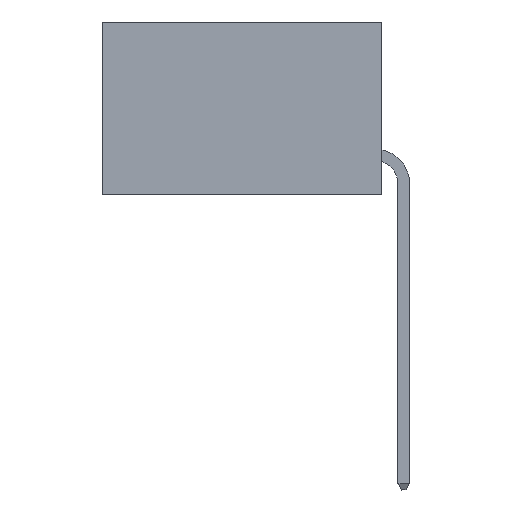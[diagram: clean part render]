
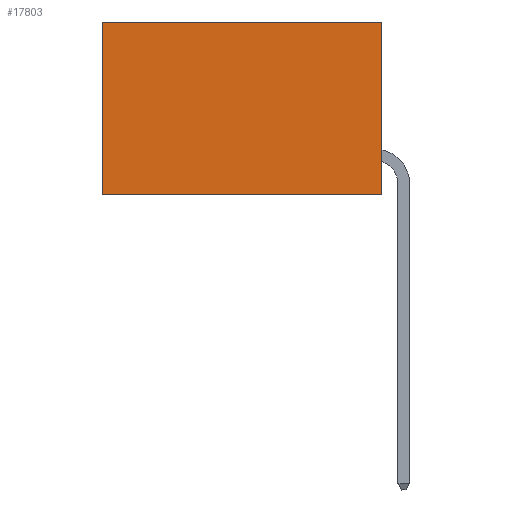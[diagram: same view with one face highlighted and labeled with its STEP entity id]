
A CAD part, left-side view. The second image highlights one B-rep face of the part: STEP entity #17803.
In plain terms, the highlighted planar face has unit normal (-1, 0, 0).
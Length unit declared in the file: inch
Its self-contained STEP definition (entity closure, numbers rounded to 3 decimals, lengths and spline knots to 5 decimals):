
#1202 = DIRECTION ( 'NONE',  ( 0., 0., -1. ) ) ;
#2442 = ORIENTED_EDGE ( 'NONE', *, *, #22988, .T. ) ;
#3109 = VERTEX_POINT ( 'NONE', #30400 ) ;
#3802 = CARTESIAN_POINT ( 'NONE',  ( 0.2875, 0., 0. ) ) ;
#4311 = VERTEX_POINT ( 'NONE', #10016 ) ;
#5636 = VECTOR ( 'NONE', #1202, 39.37008 ) ;
#6077 = ORIENTED_EDGE ( 'NONE', *, *, #27739, .F. ) ;
#6098 = VERTEX_POINT ( 'NONE', #28958 ) ;
#6115 = CARTESIAN_POINT ( 'NONE',  ( 0.2875, 0., 0. ) ) ;
#7193 = DIRECTION ( 'NONE',  ( 0., 0., -1. ) ) ;
#7658 = PLANE ( 'NONE',  #11790 ) ;
#7664 = EDGE_CURVE ( 'NONE', #16431, #3109, #23859, .T. ) ;
#9988 = ORIENTED_EDGE ( 'NONE', *, *, #7664, .T. ) ;
#10016 = CARTESIAN_POINT ( 'NONE',  ( 0.2875, 0., -0.37 ) ) ;
#10229 = DIRECTION ( 'NONE',  ( 0., 1., 0. ) ) ;
#10330 = CARTESIAN_POINT ( 'NONE',  ( 0.2875, 0., 0. ) ) ;
#10453 = EDGE_CURVE ( 'NONE', #16431, #4311, #30232, .T. ) ;
#10550 = ORIENTED_EDGE ( 'NONE', *, *, #10453, .F. ) ;
#11790 = AXIS2_PLACEMENT_3D ( 'NONE', #10330, #23190, #7193 ) ;
#11953 = VECTOR ( 'NONE', #15576, 39.37008 ) ;
#12030 = EDGE_LOOP ( 'NONE', ( #2442, #6077, #10550, #9988 ) ) ;
#12722 = CARTESIAN_POINT ( 'NONE',  ( 0.2875, 0., 0. ) ) ;
#15065 = VECTOR ( 'NONE', #10229, 39.37008 ) ;
#15576 = DIRECTION ( 'NONE',  ( 0., 0., -1. ) ) ;
#16431 = VERTEX_POINT ( 'NONE', #12722 ) ;
#17803 = ADVANCED_FACE ( 'NONE', ( #21502 ), #7658, .F. ) ;
#19664 = VECTOR ( 'NONE', #22470, 39.37008 ) ;
#21502 = FACE_OUTER_BOUND ( 'NONE', #12030, .T. ) ;
#22470 = DIRECTION ( 'NONE',  ( 0., 1., 0. ) ) ;
#22988 = EDGE_CURVE ( 'NONE', #3109, #6098, #23284, .T. ) ;
#22996 = LINE ( 'NONE', #23208, #15065 ) ;
#23190 = DIRECTION ( 'NONE',  ( 1., 0., 0. ) ) ;
#23208 = CARTESIAN_POINT ( 'NONE',  ( 0.2875, 0., -0.37 ) ) ;
#23284 = LINE ( 'NONE', #24077, #11953 ) ;
#23859 = LINE ( 'NONE', #6115, #19664 ) ;
#24077 = CARTESIAN_POINT ( 'NONE',  ( 0.2875, 0.6, 0. ) ) ;
#27739 = EDGE_CURVE ( 'NONE', #4311, #6098, #22996, .T. ) ;
#28958 = CARTESIAN_POINT ( 'NONE',  ( 0.2875, 0.6, -0.37 ) ) ;
#30232 = LINE ( 'NONE', #3802, #5636 ) ;
#30400 = CARTESIAN_POINT ( 'NONE',  ( 0.2875, 0.6, 0. ) ) ;
